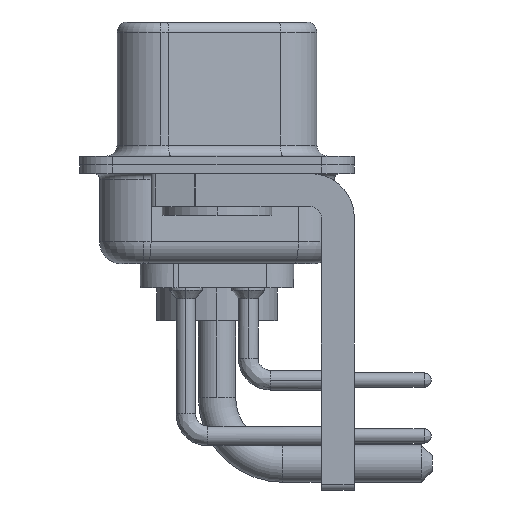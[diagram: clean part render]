
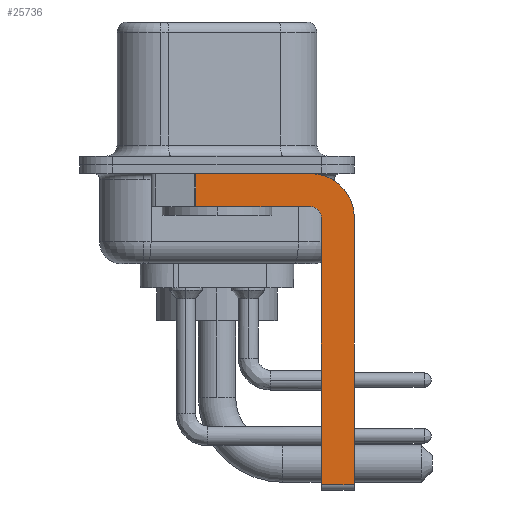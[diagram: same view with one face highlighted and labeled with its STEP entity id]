
A CAD part, left-side view. The second image highlights one B-rep face of the part: STEP entity #25736.
In plain terms, the highlighted planar face has unit normal (-1, 0, 0).
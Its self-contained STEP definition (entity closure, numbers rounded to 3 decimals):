
#402 = LINE ( 'NONE', #11037, #9222 ) ;
#802 = DIRECTION ( 'NONE',  ( 0., 0., -1. ) ) ;
#813 = CIRCLE ( 'NONE', #5988, 0.5 ) ;
#880 = EDGE_CURVE ( 'NONE', #3205, #13362, #2823, .T. ) ;
#1426 = CARTESIAN_POINT ( 'NONE',  ( -2.9, -6.25, -2.4 ) ) ;
#2006 = ORIENTED_EDGE ( 'NONE', *, *, #16969, .F. ) ;
#2469 = CARTESIAN_POINT ( 'NONE',  ( -2.9, -4.75, -14.55 ) ) ;
#2823 = LINE ( 'NONE', #19146, #20750 ) ;
#3205 = VERTEX_POINT ( 'NONE', #7090 ) ;
#3669 = CARTESIAN_POINT ( 'NONE',  ( -2.9, -4.25, -1.9 ) ) ;
#4123 = DIRECTION ( 'NONE',  ( 0., 0., 1. ) ) ;
#5331 = DIRECTION ( 'NONE',  ( 0., 0., 1. ) ) ;
#5726 = VECTOR ( 'NONE', #22266, 1000. ) ;
#5736 = CARTESIAN_POINT ( 'NONE',  ( -2.9, -4.75, -14.8 ) ) ;
#5760 = CARTESIAN_POINT ( 'NONE',  ( -2.9, 3., -0.4 ) ) ;
#5978 = DIRECTION ( 'NONE',  ( 0., 0., -1. ) ) ;
#5988 = AXIS2_PLACEMENT_3D ( 'NONE', #24197, #18392, #4123 ) ;
#6065 = VERTEX_POINT ( 'NONE', #6188 ) ;
#6188 = CARTESIAN_POINT ( 'NONE',  ( -2.9, -4.25, -0.4 ) ) ;
#6238 = CARTESIAN_POINT ( 'NONE',  ( -2.9, -6.25, -14.55 ) ) ;
#6512 = ORIENTED_EDGE ( 'NONE', *, *, #7547, .T. ) ;
#7088 = CARTESIAN_POINT ( 'NONE',  ( -2.9, -4.25, -2.4 ) ) ;
#7090 = CARTESIAN_POINT ( 'NONE',  ( -2.9, 0.978, -0.4 ) ) ;
#7547 = EDGE_CURVE ( 'NONE', #17444, #7644, #24295, .T. ) ;
#7644 = VERTEX_POINT ( 'NONE', #6238 ) ;
#7648 = ORIENTED_EDGE ( 'NONE', *, *, #8699, .F. ) ;
#7673 = EDGE_LOOP ( 'NONE', ( #2006, #14843, #8635, #23882, #7648, #6512, #22922, #11442 ) ) ;
#8122 = CARTESIAN_POINT ( 'NONE',  ( -2.9, -4.25, -14.55 ) ) ;
#8635 = ORIENTED_EDGE ( 'NONE', *, *, #16752, .F. ) ;
#8699 = EDGE_CURVE ( 'NONE', #17444, #22252, #13961, .T. ) ;
#8898 = CARTESIAN_POINT ( 'NONE',  ( -2.9, -6.25, -2.4 ) ) ;
#9222 = VECTOR ( 'NONE', #14972, 1000. ) ;
#10093 = VECTOR ( 'NONE', #5331, 1000. ) ;
#11037 = CARTESIAN_POINT ( 'NONE',  ( -2.9, -4.25, -1.9 ) ) ;
#11442 = ORIENTED_EDGE ( 'NONE', *, *, #25646, .F. ) ;
#11488 = CIRCLE ( 'NONE', #15364, 2. ) ;
#11917 = DIRECTION ( 'NONE',  ( 1., 0., 0. ) ) ;
#12041 = CARTESIAN_POINT ( 'NONE',  ( -2.9, -4.75, -2.4 ) ) ;
#12401 = CARTESIAN_POINT ( 'NONE',  ( -2.9, 0.978, -1.9 ) ) ;
#13362 = VERTEX_POINT ( 'NONE', #12401 ) ;
#13753 = EDGE_CURVE ( 'NONE', #22252, #14074, #813, .T. ) ;
#13961 = LINE ( 'NONE', #5736, #10093 ) ;
#14074 = VERTEX_POINT ( 'NONE', #3669 ) ;
#14843 = ORIENTED_EDGE ( 'NONE', *, *, #880, .T. ) ;
#14972 = DIRECTION ( 'NONE',  ( 0., 1., 0. ) ) ;
#15319 = DIRECTION ( 'NONE',  ( 0., 0., -1. ) ) ;
#15364 = AXIS2_PLACEMENT_3D ( 'NONE', #7088, #21633, #15319 ) ;
#16511 = CARTESIAN_POINT ( 'NONE',  ( -2.9, -4.25, -2.4 ) ) ;
#16752 = EDGE_CURVE ( 'NONE', #14074, #13362, #402, .T. ) ;
#16969 = EDGE_CURVE ( 'NONE', #3205, #6065, #20596, .T. ) ;
#17099 = AXIS2_PLACEMENT_3D ( 'NONE', #16511, #11917, #5978 ) ;
#17444 = VERTEX_POINT ( 'NONE', #2469 ) ;
#18066 = EDGE_CURVE ( 'NONE', #18765, #7644, #25201, .T. ) ;
#18392 = DIRECTION ( 'NONE',  ( -1., 0., 0. ) ) ;
#18765 = VERTEX_POINT ( 'NONE', #1426 ) ;
#19146 = CARTESIAN_POINT ( 'NONE',  ( -2.9, 0.978, -1.9 ) ) ;
#19192 = VECTOR ( 'NONE', #23175, 1000. ) ;
#20424 = FACE_OUTER_BOUND ( 'NONE', #7673, .T. ) ;
#20596 = LINE ( 'NONE', #5760, #22576 ) ;
#20750 = VECTOR ( 'NONE', #802, 1000. ) ;
#21633 = DIRECTION ( 'NONE',  ( 1., 0., 0. ) ) ;
#22252 = VERTEX_POINT ( 'NONE', #12041 ) ;
#22266 = DIRECTION ( 'NONE',  ( 0., -1., 0. ) ) ;
#22576 = VECTOR ( 'NONE', #26518, 1000. ) ;
#22922 = ORIENTED_EDGE ( 'NONE', *, *, #18066, .F. ) ;
#23175 = DIRECTION ( 'NONE',  ( 0., 0., -1. ) ) ;
#23882 = ORIENTED_EDGE ( 'NONE', *, *, #13753, .F. ) ;
#24197 = CARTESIAN_POINT ( 'NONE',  ( -2.9, -4.25, -2.4 ) ) ;
#24295 = LINE ( 'NONE', #8122, #5726 ) ;
#24322 = PLANE ( 'NONE',  #17099 ) ;
#25201 = LINE ( 'NONE', #8898, #19192 ) ;
#25646 = EDGE_CURVE ( 'NONE', #6065, #18765, #11488, .T. ) ;
#25736 = ADVANCED_FACE ( 'NONE', ( #20424 ), #24322, .F. ) ;
#26518 = DIRECTION ( 'NONE',  ( 0., -1., 0. ) ) ;
